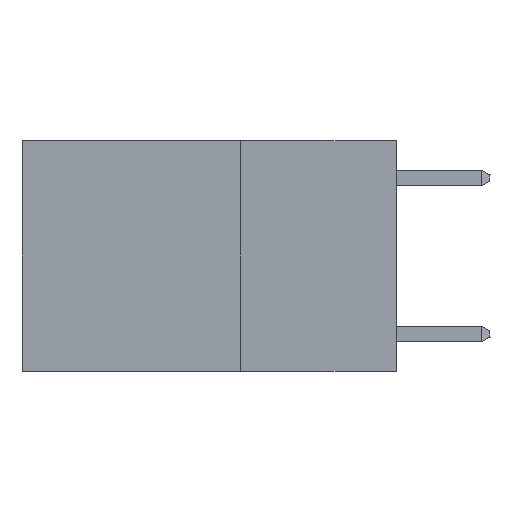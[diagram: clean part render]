
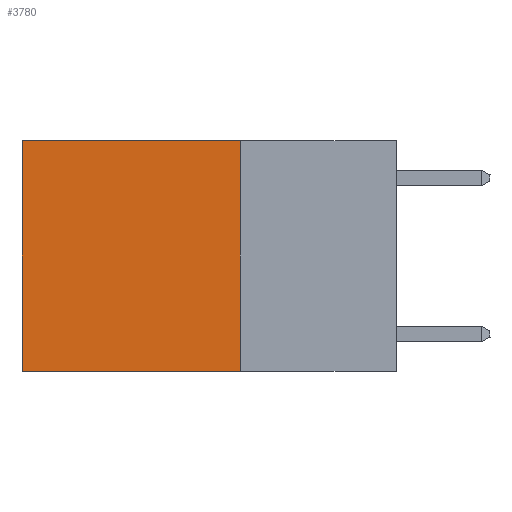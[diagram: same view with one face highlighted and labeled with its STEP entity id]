
A CAD part, left-side view. The second image highlights one B-rep face of the part: STEP entity #3780.
In plain terms, the highlighted planar face has unit normal (-1, 0, 0).
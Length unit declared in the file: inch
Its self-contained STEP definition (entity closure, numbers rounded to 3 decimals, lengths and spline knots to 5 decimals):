
#87 = CARTESIAN_POINT ( 'NONE',  ( 0.2625, 0.25, 0. ) ) ;
#218 = VERTEX_POINT ( 'NONE', #5953 ) ;
#338 = CARTESIAN_POINT ( 'NONE',  ( 0.2625, 0.25, 0. ) ) ;
#648 = CARTESIAN_POINT ( 'NONE',  ( 0.2625, 0.25, -0.37 ) ) ;
#702 = AXIS2_PLACEMENT_3D ( 'NONE', #87, #952, #9370 ) ;
#764 = CARTESIAN_POINT ( 'NONE',  ( 0.2625, 0.6, -0.37 ) ) ;
#887 = FACE_OUTER_BOUND ( 'NONE', #3143, .T. ) ;
#952 = DIRECTION ( 'NONE',  ( 1., 0., 0. ) ) ;
#1200 = CARTESIAN_POINT ( 'NONE',  ( 0.2625, 0.25, 0. ) ) ;
#1319 = VERTEX_POINT ( 'NONE', #7452 ) ;
#1612 = LINE ( 'NONE', #2503, #6615 ) ;
#1752 = VECTOR ( 'NONE', #9013, 39.37008 ) ;
#2309 = EDGE_CURVE ( 'NONE', #1319, #3046, #1612, .T. ) ;
#2330 = VECTOR ( 'NONE', #9458, 39.37008 ) ;
#2503 = CARTESIAN_POINT ( 'NONE',  ( 0.2625, 0.6, 0. ) ) ;
#2918 = ORIENTED_EDGE ( 'NONE', *, *, #7085, .T. ) ;
#3046 = VERTEX_POINT ( 'NONE', #764 ) ;
#3143 = EDGE_LOOP ( 'NONE', ( #3460, #4700, #6125, #2918 ) ) ;
#3460 = ORIENTED_EDGE ( 'NONE', *, *, #2309, .T. ) ;
#3780 = ADVANCED_FACE ( 'NONE', ( #887 ), #8495, .F. ) ;
#4119 = LINE ( 'NONE', #648, #1752 ) ;
#4700 = ORIENTED_EDGE ( 'NONE', *, *, #10243, .F. ) ;
#4824 = VERTEX_POINT ( 'NONE', #5672 ) ;
#5520 = LINE ( 'NONE', #338, #2330 ) ;
#5672 = CARTESIAN_POINT ( 'NONE',  ( 0.2625, 0.25, 0. ) ) ;
#5953 = CARTESIAN_POINT ( 'NONE',  ( 0.2625, 0.25, -0.37 ) ) ;
#6125 = ORIENTED_EDGE ( 'NONE', *, *, #8812, .F. ) ;
#6615 = VECTOR ( 'NONE', #8383, 39.37008 ) ;
#7085 = EDGE_CURVE ( 'NONE', #4824, #1319, #9583, .T. ) ;
#7131 = DIRECTION ( 'NONE',  ( 0., 1., 0. ) ) ;
#7452 = CARTESIAN_POINT ( 'NONE',  ( 0.2625, 0.6, 0. ) ) ;
#8146 = VECTOR ( 'NONE', #7131, 39.37008 ) ;
#8383 = DIRECTION ( 'NONE',  ( 0., 0., -1. ) ) ;
#8495 = PLANE ( 'NONE',  #702 ) ;
#8812 = EDGE_CURVE ( 'NONE', #4824, #218, #5520, .T. ) ;
#9013 = DIRECTION ( 'NONE',  ( 0., 1., 0. ) ) ;
#9370 = DIRECTION ( 'NONE',  ( 0., 0., -1. ) ) ;
#9458 = DIRECTION ( 'NONE',  ( 0., 0., -1. ) ) ;
#9583 = LINE ( 'NONE', #1200, #8146 ) ;
#10243 = EDGE_CURVE ( 'NONE', #218, #3046, #4119, .T. ) ;
